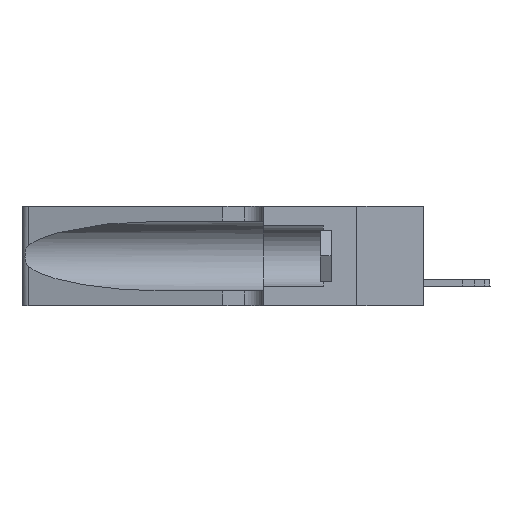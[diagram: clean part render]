
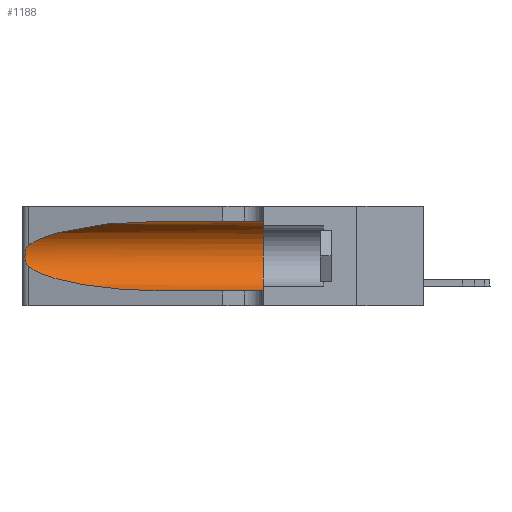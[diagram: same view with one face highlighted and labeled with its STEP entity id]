
A CAD part, left-side view. The second image highlights one B-rep face of the part: STEP entity #1188.
In plain terms, the highlighted cylindrical face has radius 3.308 mm (diameter 6.617 mm), a partial arc.
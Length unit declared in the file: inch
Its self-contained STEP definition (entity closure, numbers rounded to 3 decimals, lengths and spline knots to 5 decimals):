
#160 = CARTESIAN_POINT ( 'NONE',  ( 0.1305, 0.72297, 0.05475 ) ) ;
#842 = CARTESIAN_POINT ( 'NONE',  ( 0.2373, 1.15595, 0.28018 ) ) ;
#1188 = ADVANCED_FACE ( 'NONE', ( #2807 ), #3297, .F. ) ;
#1476 = VERTEX_POINT ( 'NONE', #7273 ) ;
#2807 = FACE_OUTER_BOUND ( 'NONE', #19761, .T. ) ;
#3297 = CYLINDRICAL_SURFACE ( 'NONE', #4604, 0.13025 ) ;
#3354 = ORIENTED_EDGE ( 'NONE', *, *, #21031, .F. ) ;
#3583 = VECTOR ( 'NONE', #8262, 39.37008 ) ;
#3669 = CARTESIAN_POINT ( 'NONE',  ( 0.25487, 1.22718, 0.22369 ) ) ;
#4604 = AXIS2_PLACEMENT_3D ( 'NONE', #12467, #21731, #24939 ) ;
#6490 = VERTEX_POINT ( 'NONE', #21016 ) ;
#6599 = CARTESIAN_POINT ( 'NONE',  ( 0.18966, 0.96281, 0.05475 ) ) ;
#6612 = CARTESIAN_POINT ( 'NONE',  ( 0.18966, 0.96281, 0.31525 ) ) ;
#7273 = CARTESIAN_POINT ( 'NONE',  ( 0.1305, 0.35, 0.05475 ) ) ;
#7486 = CIRCLE ( 'NONE', #10825, 0.13025 ) ;
#8026 = ORIENTED_EDGE ( 'NONE', *, *, #9321, .T. ) ;
#8134 = CARTESIAN_POINT ( 'NONE',  ( 0.1305, 0.72297, 0.05475 ) ) ;
#8262 = DIRECTION ( 'NONE',  ( 0., -1., 0. ) ) ;
#9301 = CARTESIAN_POINT ( 'NONE',  ( 0.25639, 1.23184, 0.21858 ) ) ;
#9321 = EDGE_CURVE ( 'NONE', #39875, #37679, #18616, .T. ) ;
#10514 = VERTEX_POINT ( 'NONE', #8134 ) ;
#10825 = AXIS2_PLACEMENT_3D ( 'NONE', #16414, #19521, #38081 ) ;
#10848 = LINE ( 'NONE', #12093, #33478 ) ;
#11084 = ORIENTED_EDGE ( 'NONE', *, *, #33531, .T. ) ;
#11182 = CARTESIAN_POINT ( 'NONE',  ( 0.1305, 1.61858, 0.31525 ) ) ;
#11786 = CARTESIAN_POINT ( 'NONE',  ( 0.25555, 1.22994, 0.2215 ) ) ;
#12093 = CARTESIAN_POINT ( 'NONE',  ( 0.1305, 1.61858, 0.05475 ) ) ;
#12467 = CARTESIAN_POINT ( 'NONE',  ( 0.1305, 1.61858, 0.185 ) ) ;
#12651 = CARTESIAN_POINT ( 'NONE',  ( 0.1305, 0.72297, 0.31525 ) ) ;
#13816 = CARTESIAN_POINT ( 'NONE',  ( 0.1305, 0.35, 0.31525 ) ) ;
#14898 = CARTESIAN_POINT ( 'NONE',  ( 0.25639, 1.23186, 0.15144 ) ) ;
#15023 = CARTESIAN_POINT ( 'NONE',  ( 0.25856, 1.23593, 0.16098 ) ) ;
#16282 = EDGE_CURVE ( 'NONE', #10514, #1476, #10848, .T. ) ;
#16414 = CARTESIAN_POINT ( 'NONE',  ( 0.1305, 0.35, 0.185 ) ) ;
#18260 = CARTESIAN_POINT ( 'NONE',  ( 0.25789, 1.23486, 0.15765 ) ) ;
#18502 = CARTESIAN_POINT ( 'NONE',  ( 0.25854, 1.2359, 0.20912 ) ) ;
#18616 =( BOUNDED_CURVE ( )  B_SPLINE_CURVE ( 3, ( #12651, #6612, #842, #3669 ),
 .UNSPECIFIED., .F., .F. ) 
 B_SPLINE_CURVE_WITH_KNOTS ( ( 4, 4 ),
 ( 1.5708, 2.84003 ),
 .UNSPECIFIED. ) 
 CURVE ( )  GEOMETRIC_REPRESENTATION_ITEM ( )  RATIONAL_B_SPLINE_CURVE ( ( 1., 0.87, 0.87, 1. ) ) 
 REPRESENTATION_ITEM ( '' )  );
#19521 = DIRECTION ( 'NONE',  ( 0., 1., 0. ) ) ;
#19619 =( BOUNDED_CURVE ( )  B_SPLINE_CURVE ( 3, ( #34002, #21776, #6599, #160 ),
 .UNSPECIFIED., .F., .F. ) 
 B_SPLINE_CURVE_WITH_KNOTS ( ( 4, 4 ),
 ( 3.44316, 4.71239 ),
 .UNSPECIFIED. ) 
 CURVE ( )  GEOMETRIC_REPRESENTATION_ITEM ( )  RATIONAL_B_SPLINE_CURVE ( ( 1., 0.87, 0.87, 1. ) ) 
 REPRESENTATION_ITEM ( '' )  );
#19761 = EDGE_LOOP ( 'NONE', ( #8026, #11084, #32624, #22596, #31893, #3354 ) ) ;
#19797 = VERTEX_POINT ( 'NONE', #13816 ) ;
#20001 = EDGE_CURVE ( 'NONE', #19797, #1476, #7486, .T. ) ;
#20941 = CARTESIAN_POINT ( 'NONE',  ( 0.26075, 1.23896, 0.178 ) ) ;
#21016 = CARTESIAN_POINT ( 'NONE',  ( 0.25487, 1.22718, 0.14631 ) ) ;
#21031 = EDGE_CURVE ( 'NONE', #39875, #19797, #39712, .T. ) ;
#21478 = CARTESIAN_POINT ( 'NONE',  ( 0.25555, 1.22993, 0.14849 ) ) ;
#21731 = DIRECTION ( 'NONE',  ( 0., -1., 0. ) ) ;
#21776 = CARTESIAN_POINT ( 'NONE',  ( 0.2373, 1.15595, 0.08982 ) ) ;
#22596 = ORIENTED_EDGE ( 'NONE', *, *, #16282, .T. ) ;
#24708 = DIRECTION ( 'NONE',  ( 0., -1., 0. ) ) ;
#24939 = DIRECTION ( 'NONE',  ( 0., 0., -1. ) ) ;
#25190 = CARTESIAN_POINT ( 'NONE',  ( 0.25487, 1.22718, 0.22369 ) ) ;
#27229 = CARTESIAN_POINT ( 'NONE',  ( 0.25487, 1.22718, 0.22369 ) ) ;
#31893 = ORIENTED_EDGE ( 'NONE', *, *, #20001, .F. ) ;
#32624 = ORIENTED_EDGE ( 'NONE', *, *, #39804, .T. ) ;
#33421 = CARTESIAN_POINT ( 'NONE',  ( 0.26075, 1.23896, 0.19203 ) ) ;
#33478 = VECTOR ( 'NONE', #24708, 39.37008 ) ;
#33531 = EDGE_CURVE ( 'NONE', #37679, #6490, #37099, .T. ) ;
#34002 = CARTESIAN_POINT ( 'NONE',  ( 0.25487, 1.22718, 0.14631 ) ) ;
#36552 = CARTESIAN_POINT ( 'NONE',  ( 0.26018, 1.23835, 0.19895 ) ) ;
#36678 = CARTESIAN_POINT ( 'NONE',  ( 0.26017, 1.23833, 0.17102 ) ) ;
#36934 = CARTESIAN_POINT ( 'NONE',  ( 0.25787, 1.23484, 0.2124 ) ) ;
#37099 = B_SPLINE_CURVE_WITH_KNOTS ( 'NONE', 3,
 ( #27229, #11786, #9301, #36934, #18502, #36552, #33421, #20941, #36678, #15023, #18260, #14898, #21478, #39672 ),
 .UNSPECIFIED., .F., .F.,
 ( 4, 2, 2, 2, 2, 2, 4 ),
 ( 0., 0.00027, 0.00053, 0.00107, 0.0016, 0.00187, 0.00214 ),
 .UNSPECIFIED. ) ;
#37679 = VERTEX_POINT ( 'NONE', #25190 ) ;
#38081 = DIRECTION ( 'NONE',  ( 0., 0., 1. ) ) ;
#39672 = CARTESIAN_POINT ( 'NONE',  ( 0.25487, 1.22718, 0.14631 ) ) ;
#39712 = LINE ( 'NONE', #11182, #3583 ) ;
#39804 = EDGE_CURVE ( 'NONE', #6490, #10514, #19619, .T. ) ;
#39875 = VERTEX_POINT ( 'NONE', #39879 ) ;
#39879 = CARTESIAN_POINT ( 'NONE',  ( 0.1305, 0.72297, 0.31525 ) ) ;
